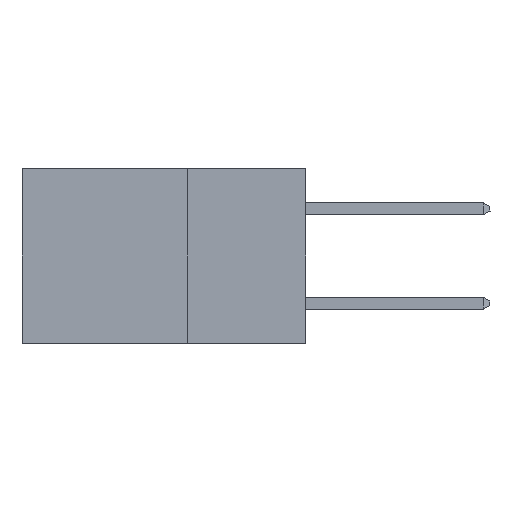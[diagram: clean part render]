
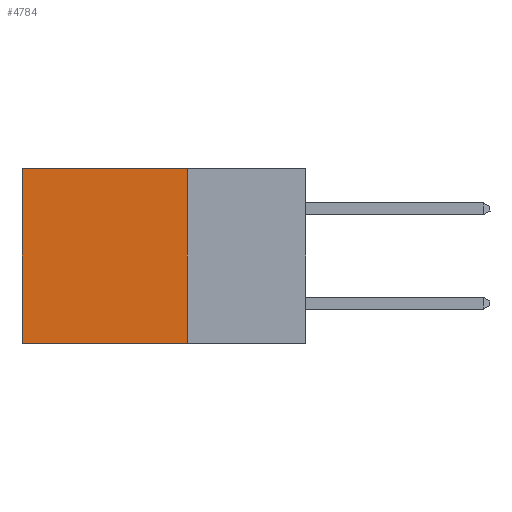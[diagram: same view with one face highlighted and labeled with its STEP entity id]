
A CAD part, left-side view. The second image highlights one B-rep face of the part: STEP entity #4784.
In plain terms, the highlighted planar face has unit normal (-1, 0, 0).
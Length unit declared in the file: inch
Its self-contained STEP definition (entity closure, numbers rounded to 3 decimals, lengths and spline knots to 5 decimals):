
#201 = LINE ( 'NONE', #3821, #8691 ) ;
#397 = CARTESIAN_POINT ( 'NONE',  ( 0.298, 0.25, -0.37 ) ) ;
#772 = ORIENTED_EDGE ( 'NONE', *, *, #2805, .T. ) ;
#870 = EDGE_CURVE ( 'NONE', #3937, #5722, #7801, .T. ) ;
#987 = EDGE_LOOP ( 'NONE', ( #772, #6587, #8084, #8675 ) ) ;
#1701 = PLANE ( 'NONE',  #9972 ) ;
#1737 = CARTESIAN_POINT ( 'NONE',  ( 0.298, 0.25, 0. ) ) ;
#1818 = CARTESIAN_POINT ( 'NONE',  ( 0.298, 0.25, -0.37 ) ) ;
#2436 = DIRECTION ( 'NONE',  ( 0., 1., 0. ) ) ;
#2805 = EDGE_CURVE ( 'NONE', #9957, #7817, #8137, .T. ) ;
#3098 = DIRECTION ( 'NONE',  ( 0., 0., -1. ) ) ;
#3419 = VECTOR ( 'NONE', #3608, 39.37008 ) ;
#3512 = CARTESIAN_POINT ( 'NONE',  ( 0.298, 0.6, -0.37 ) ) ;
#3608 = DIRECTION ( 'NONE',  ( 0., 1., 0. ) ) ;
#3821 = CARTESIAN_POINT ( 'NONE',  ( 0.298, 0.25, 0. ) ) ;
#3929 = CARTESIAN_POINT ( 'NONE',  ( 0.298, 0.6, 0. ) ) ;
#3937 = VERTEX_POINT ( 'NONE', #6499 ) ;
#4140 = DIRECTION ( 'NONE',  ( 0., 0., -1. ) ) ;
#4784 = ADVANCED_FACE ( 'NONE', ( #9266 ), #1701, .F. ) ;
#4990 = DIRECTION ( 'NONE',  ( 1., 0., 0. ) ) ;
#5067 = VECTOR ( 'NONE', #5202, 39.37008 ) ;
#5202 = DIRECTION ( 'NONE',  ( 0., 0., -1. ) ) ;
#5722 = VERTEX_POINT ( 'NONE', #1818 ) ;
#6054 = VECTOR ( 'NONE', #3098, 39.37008 ) ;
#6286 = CARTESIAN_POINT ( 'NONE',  ( 0.298, 0.25, 0. ) ) ;
#6499 = CARTESIAN_POINT ( 'NONE',  ( 0.298, 0.25, 0. ) ) ;
#6587 = ORIENTED_EDGE ( 'NONE', *, *, #7076, .F. ) ;
#7076 = EDGE_CURVE ( 'NONE', #5722, #7817, #9356, .T. ) ;
#7700 = EDGE_CURVE ( 'NONE', #3937, #9957, #201, .T. ) ;
#7801 = LINE ( 'NONE', #6286, #5067 ) ;
#7817 = VERTEX_POINT ( 'NONE', #3512 ) ;
#8084 = ORIENTED_EDGE ( 'NONE', *, *, #870, .F. ) ;
#8137 = LINE ( 'NONE', #3929, #6054 ) ;
#8675 = ORIENTED_EDGE ( 'NONE', *, *, #7700, .T. ) ;
#8691 = VECTOR ( 'NONE', #2436, 39.37008 ) ;
#8768 = CARTESIAN_POINT ( 'NONE',  ( 0.298, 0.6, 0. ) ) ;
#9266 = FACE_OUTER_BOUND ( 'NONE', #987, .T. ) ;
#9356 = LINE ( 'NONE', #397, #3419 ) ;
#9957 = VERTEX_POINT ( 'NONE', #8768 ) ;
#9972 = AXIS2_PLACEMENT_3D ( 'NONE', #1737, #4990, #4140 ) ;
